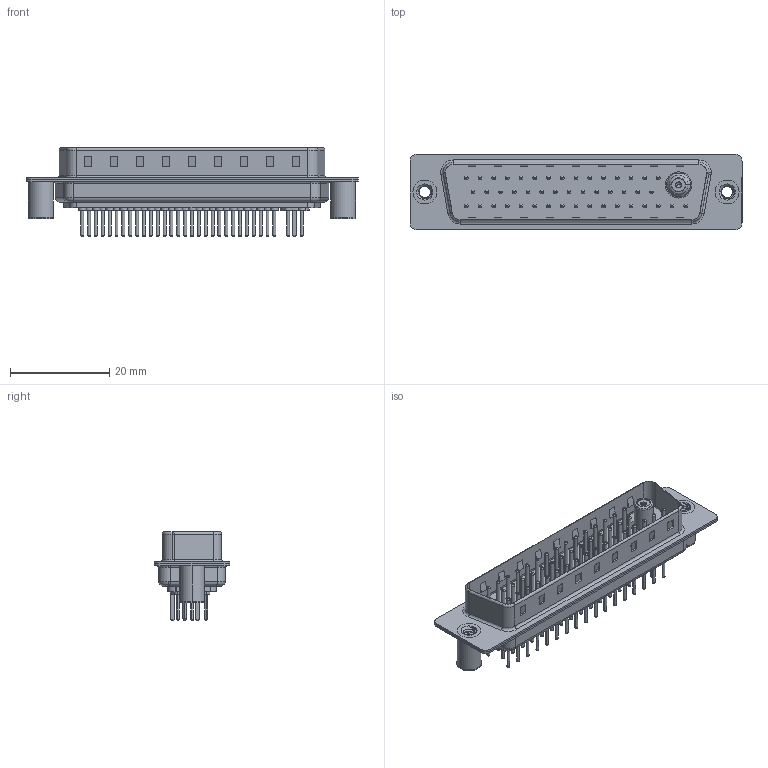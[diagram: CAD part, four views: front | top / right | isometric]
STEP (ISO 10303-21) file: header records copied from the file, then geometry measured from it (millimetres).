
FILE_DESCRIPTION (( 'STEP AP203' ), '1' );
FILE_NAME ('627-47W1624-7T3.STEP', '2019-06-20T18:04:57', ( '' ), ( '' ), 'SwSTEP 2.0', 'SolidWorks 2016', '' );
FILE_SCHEMA (( 'CONFIG_CONTROL_DESIGN' ));
Length unit declared in the file: millimetre
Products named in the file (14): 627Combo Shell Front_50 Contacts; 627Combo Contact Row 1_24; Locking Collar; 627-47W1624-7T3; 627Combo Contact Row 2_24; 627Combo Contact Row 3_24; Insulator Socket; 627Combo Shell Rear_50 Contacts; Insulator Socket 2; 627Combo Threaded Board Spacer_3; Co-Ax Jack Assy_St; Co-Ax Jack_Straight PC Tail; Socket_Str; 627Combo Housing_47W1
Assembly tree (57 placements, depth 3):
  627-47W1624-7T3
    627Combo Housing_47W1
    627Combo Shell Rear_50 Contacts
    627Combo Shell Front_50 Contacts
    627Combo Threaded Board Spacer_3  x2
    Co-Ax Jack Assy_St
      Co-Ax Jack_Straight PC Tail
      Insulator Socket
      Insulator Socket 2
      Locking Collar
      Socket_Str
    627Combo Contact Row 1_24  x15
    627Combo Contact Row 2_24  x14
    627Combo Contact Row 3_24  x17
Bounding box: 67 x 15.3 x 17.9 mm (x, y, z)
Volume: 4670.7 mm3; surface area: 11438.2 mm2
Topology: 56 solids, 56 shells, 2259 faces, 4794 edges, 2896 vertices
Faces by surface type: cylinder 856, torus 794, plane 572, cone 27, bspline 8, sphere 2
Entity records: 32630 total; most frequent: CARTESIAN_POINT 6539, DIRECTION 5342, ORIENTED_EDGE 4514, EDGE_CURVE 2257, AXIS2_PLACEMENT_3D 2142, VERTEX_POINT 1443, EDGE_LOOP 1236, CIRCLE 1124
